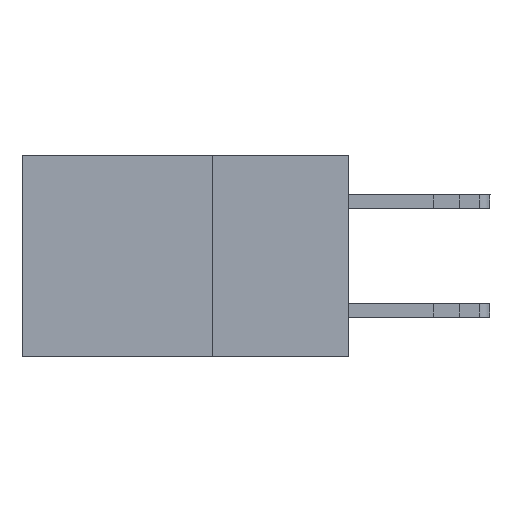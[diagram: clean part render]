
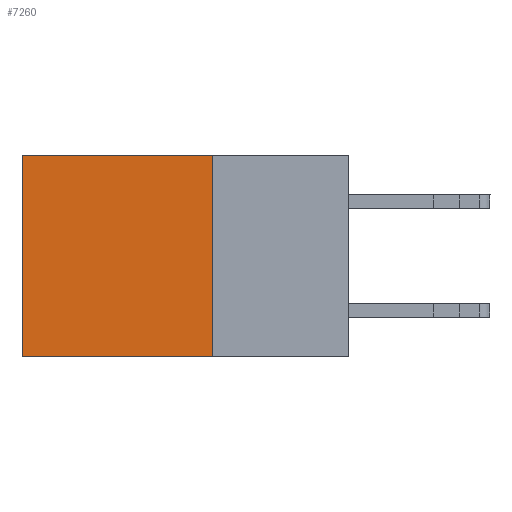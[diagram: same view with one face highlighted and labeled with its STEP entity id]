
A CAD part, left-side view. The second image highlights one B-rep face of the part: STEP entity #7260.
In plain terms, the highlighted planar face has unit normal (-1, 0, 0).
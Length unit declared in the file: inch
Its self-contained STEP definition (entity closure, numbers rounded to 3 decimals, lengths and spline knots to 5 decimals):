
#1115 = EDGE_CURVE ( 'NONE', #12337, #4671, #11984, .T. ) ;
#1910 = DIRECTION ( 'NONE',  ( 1., 0., 0. ) ) ;
#3118 = EDGE_LOOP ( 'NONE', ( #12584, #10967, #15330, #6026 ) ) ;
#4027 = LINE ( 'NONE', #7489, #6418 ) ;
#4652 = VECTOR ( 'NONE', #6627, 39.37008 ) ;
#4661 = FACE_OUTER_BOUND ( 'NONE', #3118, .T. ) ;
#4671 = VERTEX_POINT ( 'NONE', #13211 ) ;
#5555 = CARTESIAN_POINT ( 'NONE',  ( 0.298, 0.25, 0. ) ) ;
#6026 = ORIENTED_EDGE ( 'NONE', *, *, #1115, .T. ) ;
#6192 = DIRECTION ( 'NONE',  ( 0., 0., -1. ) ) ;
#6418 = VECTOR ( 'NONE', #11593, 39.37008 ) ;
#6448 = EDGE_CURVE ( 'NONE', #12337, #17648, #13291, .T. ) ;
#6627 = DIRECTION ( 'NONE',  ( 0., 1., 0. ) ) ;
#6663 = DIRECTION ( 'NONE',  ( 0., 0., -1. ) ) ;
#7260 = ADVANCED_FACE ( 'NONE', ( #4661 ), #15734, .F. ) ;
#7489 = CARTESIAN_POINT ( 'NONE',  ( 0.298, 0.6, 0. ) ) ;
#9582 = VECTOR ( 'NONE', #6663, 39.37008 ) ;
#9932 = AXIS2_PLACEMENT_3D ( 'NONE', #12976, #1910, #6192 ) ;
#10658 = CARTESIAN_POINT ( 'NONE',  ( 0.298, 0.25, -0.37 ) ) ;
#10854 = CARTESIAN_POINT ( 'NONE',  ( 0.298, 0.25, 0. ) ) ;
#10967 = ORIENTED_EDGE ( 'NONE', *, *, #15482, .F. ) ;
#11593 = DIRECTION ( 'NONE',  ( 0., 0., -1. ) ) ;
#11876 = VERTEX_POINT ( 'NONE', #17121 ) ;
#11984 = LINE ( 'NONE', #5555, #4652 ) ;
#11986 = LINE ( 'NONE', #10658, #14075 ) ;
#12337 = VERTEX_POINT ( 'NONE', #17103 ) ;
#12584 = ORIENTED_EDGE ( 'NONE', *, *, #16862, .T. ) ;
#12976 = CARTESIAN_POINT ( 'NONE',  ( 0.298, 0.25, 0. ) ) ;
#13211 = CARTESIAN_POINT ( 'NONE',  ( 0.298, 0.6, 0. ) ) ;
#13291 = LINE ( 'NONE', #10854, #9582 ) ;
#14075 = VECTOR ( 'NONE', #16101, 39.37008 ) ;
#15330 = ORIENTED_EDGE ( 'NONE', *, *, #6448, .F. ) ;
#15482 = EDGE_CURVE ( 'NONE', #17648, #11876, #11986, .T. ) ;
#15734 = PLANE ( 'NONE',  #9932 ) ;
#16101 = DIRECTION ( 'NONE',  ( 0., 1., 0. ) ) ;
#16285 = CARTESIAN_POINT ( 'NONE',  ( 0.298, 0.25, -0.37 ) ) ;
#16862 = EDGE_CURVE ( 'NONE', #4671, #11876, #4027, .T. ) ;
#17103 = CARTESIAN_POINT ( 'NONE',  ( 0.298, 0.25, 0. ) ) ;
#17121 = CARTESIAN_POINT ( 'NONE',  ( 0.298, 0.6, -0.37 ) ) ;
#17648 = VERTEX_POINT ( 'NONE', #16285 ) ;
